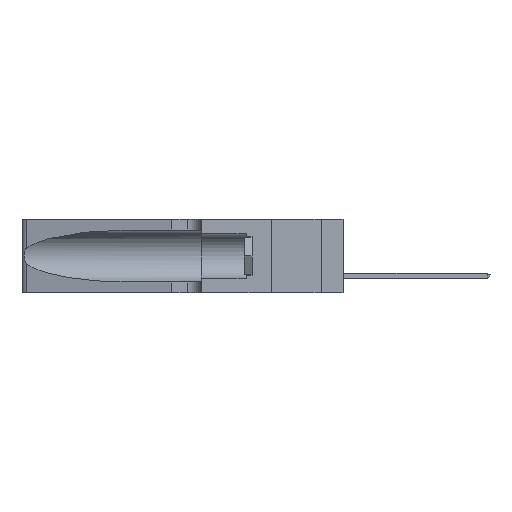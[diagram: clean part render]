
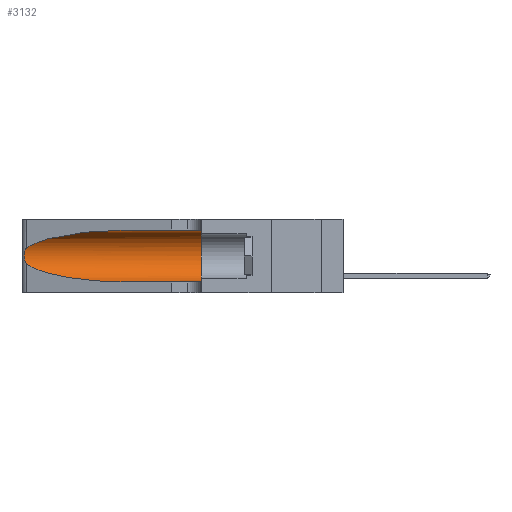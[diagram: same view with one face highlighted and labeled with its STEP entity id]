
A CAD part, left-side view. The second image highlights one B-rep face of the part: STEP entity #3132.
In plain terms, the highlighted cylindrical face has radius 3.308 mm (diameter 6.617 mm), a partial arc.
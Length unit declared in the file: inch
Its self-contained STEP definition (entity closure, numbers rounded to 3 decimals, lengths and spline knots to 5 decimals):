
#545 = ORIENTED_EDGE ( 'NONE', *, *, #4062, .T. ) ;
#709 = CARTESIAN_POINT ( 'NONE',  ( 0.1305, 0.35, 0.05475 ) ) ;
#1380 = CARTESIAN_POINT ( 'NONE',  ( 0.26018, 1.23835, 0.19895 ) ) ;
#1436 = ORIENTED_EDGE ( 'NONE', *, *, #39940, .T. ) ;
#1684 = CARTESIAN_POINT ( 'NONE',  ( 0.25555, 1.22993, 0.14849 ) ) ;
#2243 = EDGE_CURVE ( 'NONE', #16766, #37385, #29408, .T. ) ;
#2921 = CIRCLE ( 'NONE', #35102, 0.13025 ) ;
#3132 = ADVANCED_FACE ( 'NONE', ( #24116 ), #4915, .F. ) ;
#3704 = DIRECTION ( 'NONE',  ( 0., 0., -1. ) ) ;
#4062 = EDGE_CURVE ( 'NONE', #43328, #16766, #21443, .T. ) ;
#4915 = CYLINDRICAL_SURFACE ( 'NONE', #36762, 0.13025 ) ;
#5128 = CARTESIAN_POINT ( 'NONE',  ( 0.25639, 1.23184, 0.21858 ) ) ;
#5412 = CARTESIAN_POINT ( 'NONE',  ( 0.18966, 0.96281, 0.31525 ) ) ;
#6928 = CARTESIAN_POINT ( 'NONE',  ( 0.25487, 1.22718, 0.14631 ) ) ;
#7677 = CARTESIAN_POINT ( 'NONE',  ( 0.1305, 0.35, 0.31525 ) ) ;
#7790 =( BOUNDED_CURVE ( )  B_SPLINE_CURVE ( 3, ( #17369, #38406, #30971, #10961 ),
 .UNSPECIFIED., .F., .T. ) 
 B_SPLINE_CURVE_WITH_KNOTS ( ( 4, 4 ),
 ( 3.44316, 4.71239 ),
 .UNSPECIFIED. ) 
 CURVE ( )  GEOMETRIC_REPRESENTATION_ITEM ( )  RATIONAL_B_SPLINE_CURVE ( ( 1., 0.87, 0.87, 1. ) ) 
 REPRESENTATION_ITEM ( '' )  );
#7908 = EDGE_CURVE ( 'NONE', #43328, #39454, #35779, .T. ) ;
#8190 = VERTEX_POINT ( 'NONE', #38349 ) ;
#9597 = VECTOR ( 'NONE', #30262, 39.37008 ) ;
#9872 = CARTESIAN_POINT ( 'NONE',  ( 0.1305, 0.72297, 0.31525 ) ) ;
#9981 = EDGE_CURVE ( 'NONE', #8190, #34831, #13231, .T. ) ;
#10961 = CARTESIAN_POINT ( 'NONE',  ( 0.1305, 0.72297, 0.05475 ) ) ;
#11105 = ORIENTED_EDGE ( 'NONE', *, *, #2243, .T. ) ;
#11877 = CARTESIAN_POINT ( 'NONE',  ( 0.26017, 1.23833, 0.17102 ) ) ;
#13095 = CARTESIAN_POINT ( 'NONE',  ( 0.1305, 1.61858, 0.05475 ) ) ;
#13209 = ORIENTED_EDGE ( 'NONE', *, *, #9981, .T. ) ;
#13231 = LINE ( 'NONE', #13095, #29226 ) ;
#15156 = CARTESIAN_POINT ( 'NONE',  ( 0.25789, 1.23486, 0.15765 ) ) ;
#16561 = CARTESIAN_POINT ( 'NONE',  ( 0.25487, 1.22718, 0.22369 ) ) ;
#16766 = VERTEX_POINT ( 'NONE', #16561 ) ;
#17369 = CARTESIAN_POINT ( 'NONE',  ( 0.25487, 1.22718, 0.14631 ) ) ;
#17421 = CARTESIAN_POINT ( 'NONE',  ( 0.1305, 1.61858, 0.185 ) ) ;
#19000 = CARTESIAN_POINT ( 'NONE',  ( 0.25487, 1.22718, 0.22369 ) ) ;
#21443 =( BOUNDED_CURVE ( )  B_SPLINE_CURVE ( 3, ( #29135, #5412, #26121, #33044 ),
 .UNSPECIFIED., .F., .F. ) 
 B_SPLINE_CURVE_WITH_KNOTS ( ( 4, 4 ),
 ( 1.5708, 2.84003 ),
 .UNSPECIFIED. ) 
 CURVE ( )  GEOMETRIC_REPRESENTATION_ITEM ( )  RATIONAL_B_SPLINE_CURVE ( ( 1., 0.87, 0.87, 1. ) ) 
 REPRESENTATION_ITEM ( '' )  );
#24116 = FACE_OUTER_BOUND ( 'NONE', #29124, .T. ) ;
#25257 = CARTESIAN_POINT ( 'NONE',  ( 0.26075, 1.23896, 0.178 ) ) ;
#26121 = CARTESIAN_POINT ( 'NONE',  ( 0.2373, 1.15595, 0.28018 ) ) ;
#29124 = EDGE_LOOP ( 'NONE', ( #545, #11105, #1436, #13209, #36127, #35906 ) ) ;
#29135 = CARTESIAN_POINT ( 'NONE',  ( 0.1305, 0.72297, 0.31525 ) ) ;
#29226 = VECTOR ( 'NONE', #43642, 39.37008 ) ;
#29408 = B_SPLINE_CURVE_WITH_KNOTS ( 'NONE', 3,
 ( #19000, #39309, #5128, #35881, #32171, #1380, #42705, #25257, #11877, #32026, #15156, #39012, #1684, #35731 ),
 .UNSPECIFIED., .F., .F.,
 ( 4, 2, 2, 2, 2, 2, 4 ),
 ( 0., 0.00027, 0.00053, 0.00107, 0.0016, 0.00187, 0.00214 ),
 .UNSPECIFIED. ) ;
#30262 = DIRECTION ( 'NONE',  ( 0., -1., 0. ) ) ;
#30971 = CARTESIAN_POINT ( 'NONE',  ( 0.18966, 0.96281, 0.05475 ) ) ;
#32026 = CARTESIAN_POINT ( 'NONE',  ( 0.25856, 1.23593, 0.16098 ) ) ;
#32171 = CARTESIAN_POINT ( 'NONE',  ( 0.25854, 1.2359, 0.20912 ) ) ;
#33044 = CARTESIAN_POINT ( 'NONE',  ( 0.25487, 1.22718, 0.22369 ) ) ;
#33715 = CARTESIAN_POINT ( 'NONE',  ( 0.1305, 1.61858, 0.31525 ) ) ;
#34213 = CARTESIAN_POINT ( 'NONE',  ( 0.1305, 0.35, 0.185 ) ) ;
#34831 = VERTEX_POINT ( 'NONE', #709 ) ;
#35102 = AXIS2_PLACEMENT_3D ( 'NONE', #34213, #37760, #40754 ) ;
#35731 = CARTESIAN_POINT ( 'NONE',  ( 0.25487, 1.22718, 0.14631 ) ) ;
#35779 = LINE ( 'NONE', #33715, #9597 ) ;
#35881 = CARTESIAN_POINT ( 'NONE',  ( 0.25787, 1.23484, 0.2124 ) ) ;
#35906 = ORIENTED_EDGE ( 'NONE', *, *, #7908, .F. ) ;
#36127 = ORIENTED_EDGE ( 'NONE', *, *, #40482, .F. ) ;
#36762 = AXIS2_PLACEMENT_3D ( 'NONE', #17421, #41298, #3704 ) ;
#37385 = VERTEX_POINT ( 'NONE', #6928 ) ;
#37760 = DIRECTION ( 'NONE',  ( 0., 1., 0. ) ) ;
#38349 = CARTESIAN_POINT ( 'NONE',  ( 0.1305, 0.72297, 0.05475 ) ) ;
#38406 = CARTESIAN_POINT ( 'NONE',  ( 0.2373, 1.15595, 0.08982 ) ) ;
#39012 = CARTESIAN_POINT ( 'NONE',  ( 0.25639, 1.23186, 0.15144 ) ) ;
#39309 = CARTESIAN_POINT ( 'NONE',  ( 0.25555, 1.22994, 0.2215 ) ) ;
#39454 = VERTEX_POINT ( 'NONE', #7677 ) ;
#39940 = EDGE_CURVE ( 'NONE', #37385, #8190, #7790, .T. ) ;
#40482 = EDGE_CURVE ( 'NONE', #39454, #34831, #2921, .T. ) ;
#40754 = DIRECTION ( 'NONE',  ( 0., 0., 1. ) ) ;
#41298 = DIRECTION ( 'NONE',  ( 0., -1., 0. ) ) ;
#42705 = CARTESIAN_POINT ( 'NONE',  ( 0.26075, 1.23896, 0.19203 ) ) ;
#43328 = VERTEX_POINT ( 'NONE', #9872 ) ;
#43642 = DIRECTION ( 'NONE',  ( 0., -1., 0. ) ) ;
